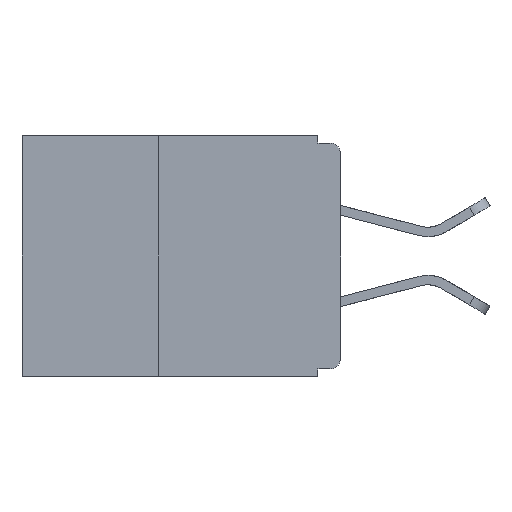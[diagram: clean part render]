
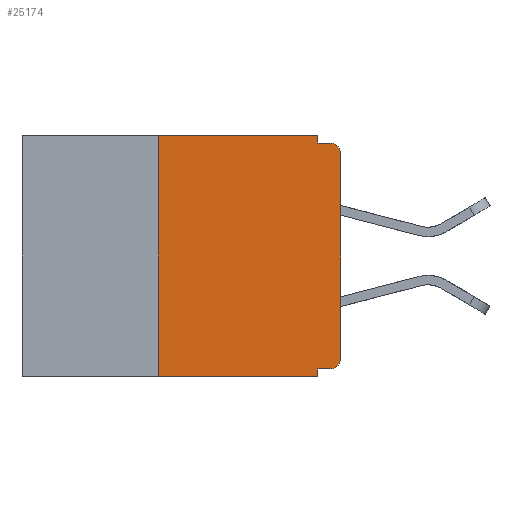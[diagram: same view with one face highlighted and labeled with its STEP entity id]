
A CAD part, left-side view. The second image highlights one B-rep face of the part: STEP entity #25174.
In plain terms, the highlighted planar face has unit normal (-1, 0, 0).
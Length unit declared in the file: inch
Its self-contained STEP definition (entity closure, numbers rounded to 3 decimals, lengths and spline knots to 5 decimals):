
#322 = CARTESIAN_POINT ( 'NONE',  ( 0., 0.015, -0.32 ) ) ;
#559 = VECTOR ( 'NONE', #22635, 39.37008 ) ;
#1078 = VECTOR ( 'NONE', #12824, 39.37008 ) ;
#1240 = VECTOR ( 'NONE', #19236, 39.37008 ) ;
#1705 = LINE ( 'NONE', #11554, #17212 ) ;
#1952 = VERTEX_POINT ( 'NONE', #10367 ) ;
#2129 = EDGE_CURVE ( 'NONE', #9260, #14595, #1705, .T. ) ;
#2230 = PLANE ( 'NONE',  #23633 ) ;
#2798 = ORIENTED_EDGE ( 'NONE', *, *, #12464, .F. ) ;
#3195 = ORIENTED_EDGE ( 'NONE', *, *, #9275, .F. ) ;
#3629 = CARTESIAN_POINT ( 'NONE',  ( 0., 0.031, 0. ) ) ;
#3943 = LINE ( 'NONE', #20422, #18740 ) ;
#4289 = DIRECTION ( 'NONE',  ( 0., 0., -1. ) ) ;
#4726 = VECTOR ( 'NONE', #21862, 39.37008 ) ;
#4851 = CARTESIAN_POINT ( 'NONE',  ( 0., 0., -0.025 ) ) ;
#5085 = DIRECTION ( 'NONE',  ( 0., -1., 0. ) ) ;
#5137 = CIRCLE ( 'NONE', #21450, 0.015 ) ;
#5158 = CARTESIAN_POINT ( 'NONE',  ( 0., 0.437, 0. ) ) ;
#5325 = CARTESIAN_POINT ( 'NONE',  ( 0., 0.437, -0.33 ) ) ;
#5921 = AXIS2_PLACEMENT_3D ( 'NONE', #9577, #23407, #11618 ) ;
#6537 = LINE ( 'NONE', #12916, #1078 ) ;
#7629 = CARTESIAN_POINT ( 'NONE',  ( 0., 0.25, 0. ) ) ;
#8859 = VERTEX_POINT ( 'NONE', #4851 ) ;
#9260 = VERTEX_POINT ( 'NONE', #22727 ) ;
#9275 = EDGE_CURVE ( 'NONE', #17668, #17968, #16743, .T. ) ;
#9286 = DIRECTION ( 'NONE',  ( 0., -1., 0. ) ) ;
#9296 = CIRCLE ( 'NONE', #5921, 0.015 ) ;
#9353 = EDGE_CURVE ( 'NONE', #1952, #8859, #25846, .T. ) ;
#9577 = CARTESIAN_POINT ( 'NONE',  ( 0., 0.015, -0.025 ) ) ;
#9682 = CARTESIAN_POINT ( 'NONE',  ( 0., 0.015, -0.305 ) ) ;
#10079 = LINE ( 'NONE', #5325, #20653 ) ;
#10367 = CARTESIAN_POINT ( 'NONE',  ( 0., 0., -0.305 ) ) ;
#10642 = EDGE_LOOP ( 'NONE', ( #12230, #11970, #2798, #3195, #17330, #11109, #23762, #11817, #17518, #23610 ) ) ;
#10706 = EDGE_CURVE ( 'NONE', #9260, #21822, #10079, .T. ) ;
#10890 = CARTESIAN_POINT ( 'NONE',  ( 0., 0., -0.01 ) ) ;
#11109 = ORIENTED_EDGE ( 'NONE', *, *, #2129, .F. ) ;
#11554 = CARTESIAN_POINT ( 'NONE',  ( 0., 0.25, -0.33 ) ) ;
#11618 = DIRECTION ( 'NONE',  ( 0., 0., -1. ) ) ;
#11725 = DIRECTION ( 'NONE',  ( 0., 0., -1. ) ) ;
#11817 = ORIENTED_EDGE ( 'NONE', *, *, #12268, .F. ) ;
#11970 = ORIENTED_EDGE ( 'NONE', *, *, #18150, .T. ) ;
#12230 = ORIENTED_EDGE ( 'NONE', *, *, #9353, .T. ) ;
#12268 = EDGE_CURVE ( 'NONE', #17057, #21822, #6537, .T. ) ;
#12464 = EDGE_CURVE ( 'NONE', #17968, #24386, #12898, .T. ) ;
#12824 = DIRECTION ( 'NONE',  ( 0., 0., -1. ) ) ;
#12898 = LINE ( 'NONE', #10890, #17546 ) ;
#12916 = CARTESIAN_POINT ( 'NONE',  ( 0., 0.031, -0.33 ) ) ;
#13668 = VERTEX_POINT ( 'NONE', #322 ) ;
#13748 = CARTESIAN_POINT ( 'NONE',  ( 0., 0.015, -0.01 ) ) ;
#14054 = EDGE_CURVE ( 'NONE', #13668, #1952, #5137, .T. ) ;
#14414 = CARTESIAN_POINT ( 'NONE',  ( 0., 0.437, 0. ) ) ;
#14595 = VERTEX_POINT ( 'NONE', #7629 ) ;
#15083 = EDGE_CURVE ( 'NONE', #14595, #17668, #16783, .T. ) ;
#16392 = DIRECTION ( 'NONE',  ( 1., 0., 0. ) ) ;
#16743 = LINE ( 'NONE', #22870, #559 ) ;
#16783 = LINE ( 'NONE', #5158, #1240 ) ;
#17034 = CARTESIAN_POINT ( 'NONE',  ( 0., 0.031, -0.01 ) ) ;
#17057 = VERTEX_POINT ( 'NONE', #23537 ) ;
#17212 = VECTOR ( 'NONE', #20242, 39.37008 ) ;
#17330 = ORIENTED_EDGE ( 'NONE', *, *, #15083, .F. ) ;
#17518 = ORIENTED_EDGE ( 'NONE', *, *, #25210, .F. ) ;
#17546 = VECTOR ( 'NONE', #9286, 39.37008 ) ;
#17668 = VERTEX_POINT ( 'NONE', #3629 ) ;
#17968 = VERTEX_POINT ( 'NONE', #17034 ) ;
#18150 = EDGE_CURVE ( 'NONE', #8859, #24386, #9296, .T. ) ;
#18740 = VECTOR ( 'NONE', #22360, 39.37008 ) ;
#19236 = DIRECTION ( 'NONE',  ( 0., -1., 0. ) ) ;
#20242 = DIRECTION ( 'NONE',  ( 0., 0., 1. ) ) ;
#20422 = CARTESIAN_POINT ( 'NONE',  ( 0., 0., -0.32 ) ) ;
#20563 = FACE_OUTER_BOUND ( 'NONE', #10642, .T. ) ;
#20653 = VECTOR ( 'NONE', #5085, 39.37008 ) ;
#21450 = AXIS2_PLACEMENT_3D ( 'NONE', #9682, #23504, #11725 ) ;
#21749 = CARTESIAN_POINT ( 'NONE',  ( 0., 0., 0. ) ) ;
#21822 = VERTEX_POINT ( 'NONE', #21885 ) ;
#21862 = DIRECTION ( 'NONE',  ( 0., 0., 1. ) ) ;
#21885 = CARTESIAN_POINT ( 'NONE',  ( 0., 0.031, -0.33 ) ) ;
#22360 = DIRECTION ( 'NONE',  ( 0., 1., 0. ) ) ;
#22635 = DIRECTION ( 'NONE',  ( 0., 0., -1. ) ) ;
#22727 = CARTESIAN_POINT ( 'NONE',  ( 0., 0.25, -0.33 ) ) ;
#22870 = CARTESIAN_POINT ( 'NONE',  ( 0., 0.031, 0. ) ) ;
#23407 = DIRECTION ( 'NONE',  ( -1., 0., 0. ) ) ;
#23504 = DIRECTION ( 'NONE',  ( -1., 0., 0. ) ) ;
#23537 = CARTESIAN_POINT ( 'NONE',  ( 0., 0.031, -0.32 ) ) ;
#23610 = ORIENTED_EDGE ( 'NONE', *, *, #14054, .T. ) ;
#23633 = AXIS2_PLACEMENT_3D ( 'NONE', #14414, #16392, #4289 ) ;
#23762 = ORIENTED_EDGE ( 'NONE', *, *, #10706, .T. ) ;
#24386 = VERTEX_POINT ( 'NONE', #13748 ) ;
#25174 = ADVANCED_FACE ( 'NONE', ( #20563 ), #2230, .F. ) ;
#25210 = EDGE_CURVE ( 'NONE', #13668, #17057, #3943, .T. ) ;
#25846 = LINE ( 'NONE', #21749, #4726 ) ;
